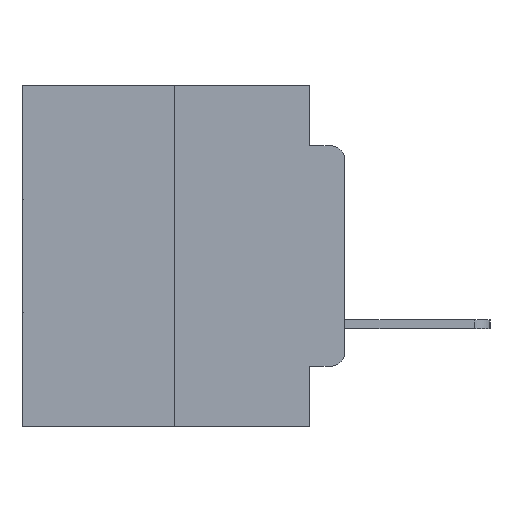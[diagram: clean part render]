
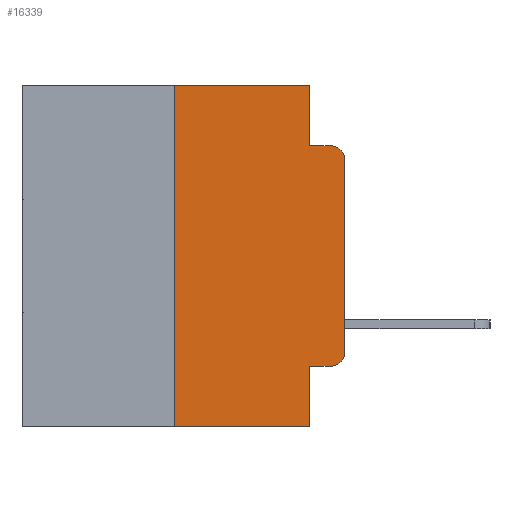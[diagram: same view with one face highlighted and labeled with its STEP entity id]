
A CAD part, left-side view. The second image highlights one B-rep face of the part: STEP entity #16339.
In plain terms, the highlighted planar face has unit normal (-1, 0, 0).
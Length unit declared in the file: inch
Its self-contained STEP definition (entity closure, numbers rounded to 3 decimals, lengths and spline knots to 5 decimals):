
#1352 = CARTESIAN_POINT ( 'NONE',  ( 0., 0.02, -0.4115 ) ) ;
#1484 = VECTOR ( 'NONE', #17041, 39.37008 ) ;
#2064 = DIRECTION ( 'NONE',  ( 0., 0., -1. ) ) ;
#2522 = DIRECTION ( 'NONE',  ( -1., 0., 0. ) ) ;
#2606 = ORIENTED_EDGE ( 'NONE', *, *, #2879, .F. ) ;
#2879 = EDGE_CURVE ( 'NONE', #14403, #23963, #9237, .T. ) ;
#2888 = LINE ( 'NONE', #9072, #24390 ) ;
#3182 = EDGE_CURVE ( 'NONE', #9554, #22136, #15123, .T. ) ;
#3381 = ORIENTED_EDGE ( 'NONE', *, *, #26895, .T. ) ;
#3577 = CARTESIAN_POINT ( 'NONE',  ( 0., 0.051, 0. ) ) ;
#4688 = ORIENTED_EDGE ( 'NONE', *, *, #24347, .T. ) ;
#4873 = AXIS2_PLACEMENT_3D ( 'NONE', #15515, #2522, #17606 ) ;
#5354 = EDGE_CURVE ( 'NONE', #20209, #15606, #16769, .T. ) ;
#5796 = VERTEX_POINT ( 'NONE', #1352 ) ;
#5875 = DIRECTION ( 'NONE',  ( 0., 0., -1. ) ) ;
#5913 = EDGE_CURVE ( 'NONE', #13420, #9554, #23768, .T. ) ;
#6224 = CARTESIAN_POINT ( 'NONE',  ( 0., 0.25, 0. ) ) ;
#6672 = CARTESIAN_POINT ( 'NONE',  ( 0., 0.473, 0. ) ) ;
#6853 = EDGE_CURVE ( 'NONE', #26881, #15606, #10137, .T. ) ;
#7365 = DIRECTION ( 'NONE',  ( 0., 0., -1. ) ) ;
#7424 = EDGE_CURVE ( 'NONE', #22136, #20209, #15623, .T. ) ;
#7642 = ORIENTED_EDGE ( 'NONE', *, *, #8393, .T. ) ;
#8393 = EDGE_CURVE ( 'NONE', #9735, #26881, #11011, .T. ) ;
#8485 = CARTESIAN_POINT ( 'NONE',  ( 0., 0.051, 0. ) ) ;
#8937 = DIRECTION ( 'NONE',  ( 1., 0., 0. ) ) ;
#8989 = CARTESIAN_POINT ( 'NONE',  ( 0., 0.473, -0.5 ) ) ;
#9072 = CARTESIAN_POINT ( 'NONE',  ( 0., 0.051, -0.4115 ) ) ;
#9237 = LINE ( 'NONE', #11596, #19545 ) ;
#9554 = VERTEX_POINT ( 'NONE', #6224 ) ;
#9735 = VERTEX_POINT ( 'NONE', #19777 ) ;
#10137 = CIRCLE ( 'NONE', #19888, 0.02 ) ;
#10430 = DIRECTION ( 'NONE',  ( 0., -1., 0. ) ) ;
#10699 = CIRCLE ( 'NONE', #4873, 0.02 ) ;
#11011 = LINE ( 'NONE', #12347, #26295 ) ;
#11106 = LINE ( 'NONE', #8989, #21266 ) ;
#11108 = DIRECTION ( 'NONE',  ( 0., -1., 0. ) ) ;
#11131 = ORIENTED_EDGE ( 'NONE', *, *, #6853, .T. ) ;
#11179 = DIRECTION ( 'NONE',  ( 0., -1., 0. ) ) ;
#11224 = VECTOR ( 'NONE', #10430, 39.37008 ) ;
#11596 = CARTESIAN_POINT ( 'NONE',  ( 0., 0.051, 0. ) ) ;
#11780 = ORIENTED_EDGE ( 'NONE', *, *, #5354, .F. ) ;
#12199 = CARTESIAN_POINT ( 'NONE',  ( 0., 0.02, -0.0885 ) ) ;
#12281 = ORIENTED_EDGE ( 'NONE', *, *, #7424, .F. ) ;
#12347 = CARTESIAN_POINT ( 'NONE',  ( 0., 0., 0. ) ) ;
#12668 = FACE_OUTER_BOUND ( 'NONE', #26868, .T. ) ;
#13420 = VERTEX_POINT ( 'NONE', #15919 ) ;
#14071 = ORIENTED_EDGE ( 'NONE', *, *, #3182, .F. ) ;
#14403 = VERTEX_POINT ( 'NONE', #21764 ) ;
#15060 = CARTESIAN_POINT ( 'NONE',  ( 0., 0.25, 0. ) ) ;
#15082 = DIRECTION ( 'NONE',  ( -1., 0., 0. ) ) ;
#15123 = LINE ( 'NONE', #18940, #24980 ) ;
#15515 = CARTESIAN_POINT ( 'NONE',  ( 0., 0.02, -0.3915 ) ) ;
#15606 = VERTEX_POINT ( 'NONE', #12199 ) ;
#15623 = LINE ( 'NONE', #3577, #25439 ) ;
#15919 = CARTESIAN_POINT ( 'NONE',  ( 0., 0.25, -0.5 ) ) ;
#16206 = CARTESIAN_POINT ( 'NONE',  ( 0., 0.051, -0.5 ) ) ;
#16294 = AXIS2_PLACEMENT_3D ( 'NONE', #6672, #8937, #23132 ) ;
#16339 = ADVANCED_FACE ( 'NONE', ( #12668 ), #19239, .F. ) ;
#16453 = DIRECTION ( 'NONE',  ( 0., 0., 1. ) ) ;
#16665 = DIRECTION ( 'NONE',  ( 0., -1., 0. ) ) ;
#16769 = LINE ( 'NONE', #18640, #11224 ) ;
#17041 = DIRECTION ( 'NONE',  ( 0., 0., 1. ) ) ;
#17370 = CARTESIAN_POINT ( 'NONE',  ( 0., 0., -0.1085 ) ) ;
#17606 = DIRECTION ( 'NONE',  ( 0., 0., -1. ) ) ;
#18507 = ORIENTED_EDGE ( 'NONE', *, *, #5913, .F. ) ;
#18640 = CARTESIAN_POINT ( 'NONE',  ( 0., 0.051, -0.0885 ) ) ;
#18940 = CARTESIAN_POINT ( 'NONE',  ( 0., 0.473, 0. ) ) ;
#19170 = ORIENTED_EDGE ( 'NONE', *, *, #21479, .T. ) ;
#19239 = PLANE ( 'NONE',  #16294 ) ;
#19545 = VECTOR ( 'NONE', #7365, 39.37008 ) ;
#19777 = CARTESIAN_POINT ( 'NONE',  ( 0., 0., -0.3915 ) ) ;
#19888 = AXIS2_PLACEMENT_3D ( 'NONE', #26806, #15082, #2064 ) ;
#20209 = VERTEX_POINT ( 'NONE', #24270 ) ;
#21266 = VECTOR ( 'NONE', #11108, 39.37008 ) ;
#21479 = EDGE_CURVE ( 'NONE', #13420, #23963, #11106, .T. ) ;
#21764 = CARTESIAN_POINT ( 'NONE',  ( 0., 0.051, -0.4115 ) ) ;
#22136 = VERTEX_POINT ( 'NONE', #8485 ) ;
#23132 = DIRECTION ( 'NONE',  ( 0., 0., -1. ) ) ;
#23768 = LINE ( 'NONE', #15060, #1484 ) ;
#23963 = VERTEX_POINT ( 'NONE', #16206 ) ;
#24270 = CARTESIAN_POINT ( 'NONE',  ( 0., 0.051, -0.0885 ) ) ;
#24347 = EDGE_CURVE ( 'NONE', #5796, #9735, #10699, .T. ) ;
#24390 = VECTOR ( 'NONE', #11179, 39.37008 ) ;
#24980 = VECTOR ( 'NONE', #16665, 39.37008 ) ;
#25439 = VECTOR ( 'NONE', #5875, 39.37008 ) ;
#26295 = VECTOR ( 'NONE', #16453, 39.37008 ) ;
#26806 = CARTESIAN_POINT ( 'NONE',  ( 0., 0.02, -0.1085 ) ) ;
#26868 = EDGE_LOOP ( 'NONE', ( #7642, #11131, #11780, #12281, #14071, #18507, #19170, #2606, #3381, #4688 ) ) ;
#26881 = VERTEX_POINT ( 'NONE', #17370 ) ;
#26895 = EDGE_CURVE ( 'NONE', #14403, #5796, #2888, .T. ) ;
